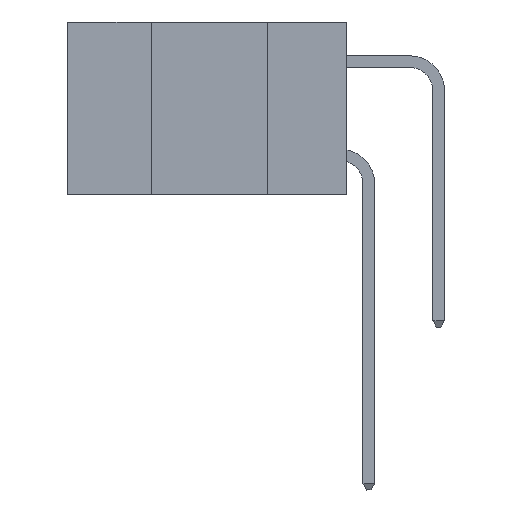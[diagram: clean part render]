
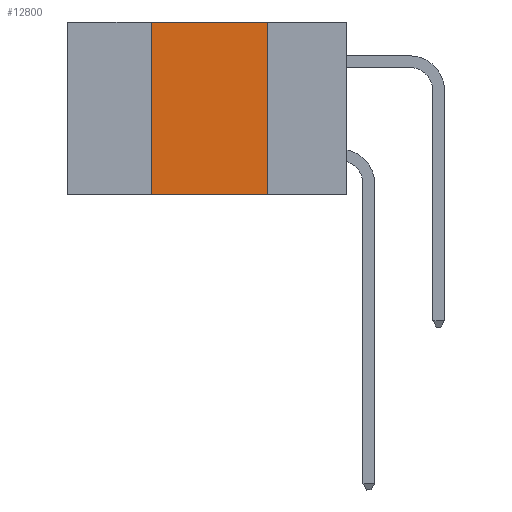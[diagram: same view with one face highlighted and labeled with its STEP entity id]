
A CAD part, left-side view. The second image highlights one B-rep face of the part: STEP entity #12800.
In plain terms, the highlighted planar face has unit normal (-1, 0, 0).
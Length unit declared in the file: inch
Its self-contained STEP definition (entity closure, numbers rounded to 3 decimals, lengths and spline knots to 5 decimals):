
#1283 = CARTESIAN_POINT ( 'NONE',  ( 0., 0.17, 0. ) ) ;
#3508 = VERTEX_POINT ( 'NONE', #14763 ) ;
#6631 = VECTOR ( 'NONE', #38433, 39.37008 ) ;
#8805 = DIRECTION ( 'NONE',  ( 0., 0., -1. ) ) ;
#10257 = ORIENTED_EDGE ( 'NONE', *, *, #36629, .F. ) ;
#10299 = EDGE_CURVE ( 'NONE', #3508, #21088, #32098, .T. ) ;
#11280 = VERTEX_POINT ( 'NONE', #20914 ) ;
#11329 = CARTESIAN_POINT ( 'NONE',  ( 0., 0.6, 0. ) ) ;
#11582 = CARTESIAN_POINT ( 'NONE',  ( 0., 0.17, -0.37 ) ) ;
#12310 = ORIENTED_EDGE ( 'NONE', *, *, #30143, .F. ) ;
#12669 = CARTESIAN_POINT ( 'NONE',  ( 0., 0.42, 0. ) ) ;
#12800 = ADVANCED_FACE ( 'NONE', ( #24067 ), #30284, .F. ) ;
#13874 = DIRECTION ( 'NONE',  ( 1., 0., 0. ) ) ;
#14032 = EDGE_LOOP ( 'NONE', ( #10257, #23788, #12310, #18097 ) ) ;
#14763 = CARTESIAN_POINT ( 'NONE',  ( 0., 0.42, 0. ) ) ;
#15037 = VECTOR ( 'NONE', #16825, 39.37008 ) ;
#16825 = DIRECTION ( 'NONE',  ( 0., 0., -1. ) ) ;
#18097 = ORIENTED_EDGE ( 'NONE', *, *, #34763, .T. ) ;
#19061 = CARTESIAN_POINT ( 'NONE',  ( 0., 0.6, 0. ) ) ;
#20914 = CARTESIAN_POINT ( 'NONE',  ( 0., 0.42, -0.37 ) ) ;
#21088 = VERTEX_POINT ( 'NONE', #38505 ) ;
#23788 = ORIENTED_EDGE ( 'NONE', *, *, #10299, .F. ) ;
#24067 = FACE_OUTER_BOUND ( 'NONE', #14032, .T. ) ;
#25422 = VERTEX_POINT ( 'NONE', #11582 ) ;
#26156 = LINE ( 'NONE', #12669, #27061 ) ;
#27061 = VECTOR ( 'NONE', #33903, 39.37008 ) ;
#27593 = AXIS2_PLACEMENT_3D ( 'NONE', #19061, #13874, #8805 ) ;
#30143 = EDGE_CURVE ( 'NONE', #11280, #3508, #26156, .T. ) ;
#30284 = PLANE ( 'NONE',  #27593 ) ;
#32098 = LINE ( 'NONE', #11329, #33012 ) ;
#32572 = DIRECTION ( 'NONE',  ( 0., -1., 0. ) ) ;
#33012 = VECTOR ( 'NONE', #32572, 39.37008 ) ;
#33903 = DIRECTION ( 'NONE',  ( 0., 0., 1. ) ) ;
#34026 = LINE ( 'NONE', #1283, #15037 ) ;
#34763 = EDGE_CURVE ( 'NONE', #11280, #25422, #38930, .T. ) ;
#35907 = CARTESIAN_POINT ( 'NONE',  ( 0., 0.6, -0.37 ) ) ;
#36629 = EDGE_CURVE ( 'NONE', #21088, #25422, #34026, .T. ) ;
#38433 = DIRECTION ( 'NONE',  ( 0., -1., 0. ) ) ;
#38505 = CARTESIAN_POINT ( 'NONE',  ( 0., 0.17, 0. ) ) ;
#38930 = LINE ( 'NONE', #35907, #6631 ) ;
